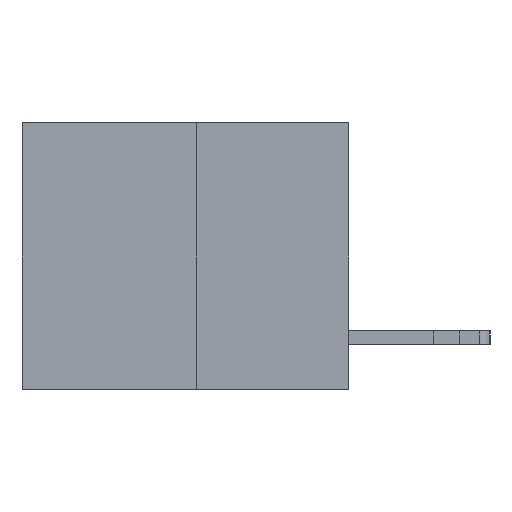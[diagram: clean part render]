
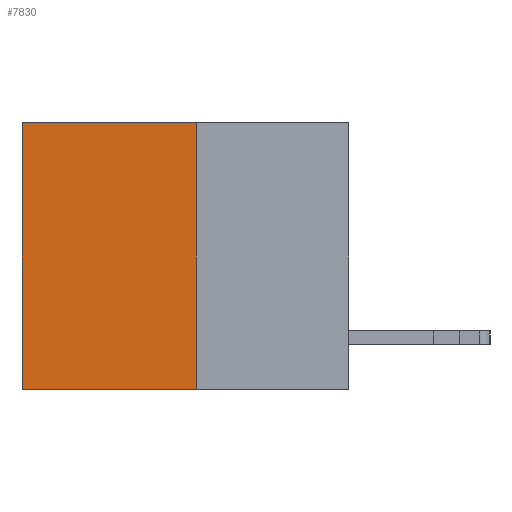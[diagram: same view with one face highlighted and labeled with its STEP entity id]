
A CAD part, left-side view. The second image highlights one B-rep face of the part: STEP entity #7830.
In plain terms, the highlighted planar face has unit normal (-1, 0, 0).
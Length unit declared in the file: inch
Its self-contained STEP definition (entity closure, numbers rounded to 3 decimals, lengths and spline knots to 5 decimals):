
#3334 = CARTESIAN_POINT ( 'NONE',  ( 0.3165, 0.6, -0.49 ) ) ;
#3610 = VERTEX_POINT ( 'NONE', #18239 ) ;
#3961 = LINE ( 'NONE', #22337, #22639 ) ;
#4788 = VECTOR ( 'NONE', #9891, 39.37008 ) ;
#5369 = AXIS2_PLACEMENT_3D ( 'NONE', #16246, #5437, #13077 ) ;
#5384 = VECTOR ( 'NONE', #20027, 39.37008 ) ;
#5437 = DIRECTION ( 'NONE',  ( 1., 0., 0. ) ) ;
#5618 = FACE_OUTER_BOUND ( 'NONE', #11233, .T. ) ;
#5769 = ORIENTED_EDGE ( 'NONE', *, *, #22839, .F. ) ;
#6773 = PLANE ( 'NONE',  #5369 ) ;
#7170 = CARTESIAN_POINT ( 'NONE',  ( 0.3165, 0.28, 0. ) ) ;
#7418 = DIRECTION ( 'NONE',  ( 0., 1., 0. ) ) ;
#7830 = ADVANCED_FACE ( 'NONE', ( #5618 ), #6773, .F. ) ;
#9891 = DIRECTION ( 'NONE',  ( 0., 1., 0. ) ) ;
#10067 = LINE ( 'NONE', #17425, #4788 ) ;
#11133 = EDGE_CURVE ( 'NONE', #22032, #3610, #3961, .T. ) ;
#11233 = EDGE_LOOP ( 'NONE', ( #21163, #5769, #18403, #20048 ) ) ;
#11457 = VERTEX_POINT ( 'NONE', #17716 ) ;
#11647 = EDGE_CURVE ( 'NONE', #11457, #16533, #14766, .T. ) ;
#13077 = DIRECTION ( 'NONE',  ( 0., 0., -1. ) ) ;
#13405 = EDGE_CURVE ( 'NONE', #22032, #11457, #16000, .T. ) ;
#14766 = LINE ( 'NONE', #23467, #5384 ) ;
#16000 = LINE ( 'NONE', #7170, #23851 ) ;
#16109 = CARTESIAN_POINT ( 'NONE',  ( 0.3165, 0.28, 0. ) ) ;
#16246 = CARTESIAN_POINT ( 'NONE',  ( 0.3165, 0.28, -0.49 ) ) ;
#16533 = VERTEX_POINT ( 'NONE', #3334 ) ;
#16836 = DIRECTION ( 'NONE',  ( 0., 0., -1. ) ) ;
#17425 = CARTESIAN_POINT ( 'NONE',  ( 0.3165, 0.28, -0.49 ) ) ;
#17716 = CARTESIAN_POINT ( 'NONE',  ( 0.3165, 0.6, 0. ) ) ;
#18239 = CARTESIAN_POINT ( 'NONE',  ( 0.3165, 0.28, -0.49 ) ) ;
#18403 = ORIENTED_EDGE ( 'NONE', *, *, #11133, .F. ) ;
#20027 = DIRECTION ( 'NONE',  ( 0., 0., -1. ) ) ;
#20048 = ORIENTED_EDGE ( 'NONE', *, *, #13405, .T. ) ;
#21163 = ORIENTED_EDGE ( 'NONE', *, *, #11647, .T. ) ;
#22032 = VERTEX_POINT ( 'NONE', #16109 ) ;
#22337 = CARTESIAN_POINT ( 'NONE',  ( 0.3165, 0.28, -0.49 ) ) ;
#22639 = VECTOR ( 'NONE', #16836, 39.37008 ) ;
#22839 = EDGE_CURVE ( 'NONE', #3610, #16533, #10067, .T. ) ;
#23467 = CARTESIAN_POINT ( 'NONE',  ( 0.3165, 0.6, -0.49 ) ) ;
#23851 = VECTOR ( 'NONE', #7418, 39.37008 ) ;
